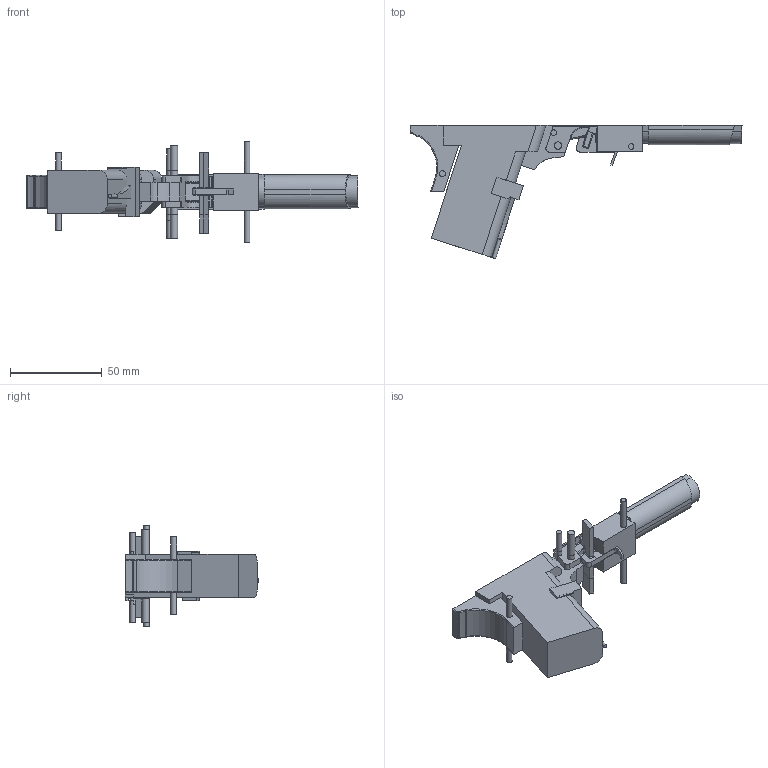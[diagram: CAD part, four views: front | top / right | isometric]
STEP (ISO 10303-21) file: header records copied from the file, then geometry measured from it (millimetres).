
FILE_DESCRIPTION(/* description */ (''),/* implementation_level */ '2;1');
FILE_NAME(/* name */ 'fmda_dd17.2_control_pocket_negative v1.step',/* time_stamp */ '2021-09-30T08:49:51-05:00',/* author */ (''),/* organization */ (''),/* preprocessor_version */ 'ST-DEVELOPER v18.1',/* originating_system */ 'Autodesk Translation Framework v10.10.0.1391',/* authorisation */ '');
FILE_SCHEMA (('AUTOMOTIVE_DESIGN { 1 0 10303 214 3 1 1 }'));
Length unit declared in the file: millimetre
Products named in the file (1): fmda_dd17.2_control_pocket_negative
Bounding box: 181 x 72.62 x 55 mm (x, y, z)
Volume: 92459.7 mm3; surface area: 23079.6 mm2
Topology: 1 solids, 1 shells, 259 faces, 671 edges, 420 vertices
Faces by surface type: plane 125, cylinder 80, bspline 27, sphere 14, torus 12, cone 1
Full cylindrical faces by diameter (mm): 2 x1, 3 x6, 3.2 x2, 4 x4
Entity records: 9045 total; most frequent: CARTESIAN_POINT 2667, ORIENTED_EDGE 1342, DIRECTION 1313, EDGE_CURVE 671, AXIS2_PLACEMENT_3D 441, LINE 431, VECTOR 431, VERTEX_POINT 420
